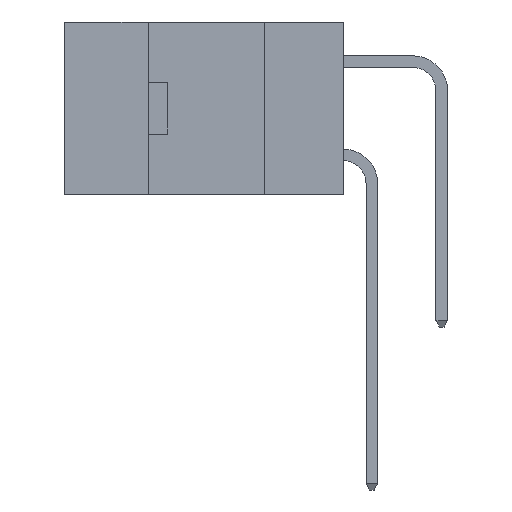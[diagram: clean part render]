
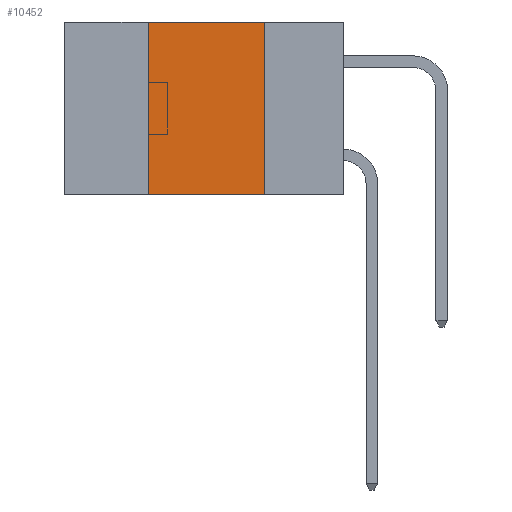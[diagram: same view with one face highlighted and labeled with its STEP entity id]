
A CAD part, left-side view. The second image highlights one B-rep face of the part: STEP entity #10452.
In plain terms, the highlighted planar face has unit normal (-1, 0, 0).
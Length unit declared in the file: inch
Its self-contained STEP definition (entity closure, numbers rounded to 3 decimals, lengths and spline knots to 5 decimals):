
#431 = LINE ( 'NONE', #9070, #17279 ) ;
#852 = EDGE_CURVE ( 'NONE', #18869, #2301, #431, .T. ) ;
#1105 = CARTESIAN_POINT ( 'NONE',  ( 0., 0.17, 0. ) ) ;
#1857 = CARTESIAN_POINT ( 'NONE',  ( 0., 0.42, -0.37 ) ) ;
#2301 = VERTEX_POINT ( 'NONE', #1105 ) ;
#2631 = DIRECTION ( 'NONE',  ( 0., 0., -1. ) ) ;
#4402 = VECTOR ( 'NONE', #2631, 39.37008 ) ;
#4627 = CARTESIAN_POINT ( 'NONE',  ( 0., 0.17, -0.37 ) ) ;
#4772 = ORIENTED_EDGE ( 'NONE', *, *, #12679, .T. ) ;
#5109 = ORIENTED_EDGE ( 'NONE', *, *, #852, .F. ) ;
#7193 = VERTEX_POINT ( 'NONE', #1857 ) ;
#7503 = ORIENTED_EDGE ( 'NONE', *, *, #10421, .F. ) ;
#7547 = DIRECTION ( 'NONE',  ( 0., 0., 1. ) ) ;
#9070 = CARTESIAN_POINT ( 'NONE',  ( 0., 0.6, 0. ) ) ;
#9170 = VECTOR ( 'NONE', #7547, 39.37008 ) ;
#10209 = LINE ( 'NONE', #24585, #4402 ) ;
#10421 = EDGE_CURVE ( 'NONE', #2301, #16166, #10209, .T. ) ;
#10452 = ADVANCED_FACE ( 'NONE', ( #21329 ), #24681, .F. ) ;
#10635 = CARTESIAN_POINT ( 'NONE',  ( 0., 0.42, 0. ) ) ;
#10643 = EDGE_CURVE ( 'NONE', #7193, #18869, #26727, .T. ) ;
#11420 = DIRECTION ( 'NONE',  ( 1., 0., 0. ) ) ;
#11490 = LINE ( 'NONE', #25446, #28327 ) ;
#12679 = EDGE_CURVE ( 'NONE', #7193, #16166, #11490, .T. ) ;
#13891 = AXIS2_PLACEMENT_3D ( 'NONE', #22478, #11420, #26831 ) ;
#16166 = VERTEX_POINT ( 'NONE', #4627 ) ;
#17279 = VECTOR ( 'NONE', #24525, 39.37008 ) ;
#17885 = EDGE_LOOP ( 'NONE', ( #7503, #5109, #23389, #4772 ) ) ;
#18869 = VERTEX_POINT ( 'NONE', #10635 ) ;
#21329 = FACE_OUTER_BOUND ( 'NONE', #17885, .T. ) ;
#22478 = CARTESIAN_POINT ( 'NONE',  ( 0., 0.6, 0. ) ) ;
#23389 = ORIENTED_EDGE ( 'NONE', *, *, #10643, .F. ) ;
#24525 = DIRECTION ( 'NONE',  ( 0., -1., 0. ) ) ;
#24585 = CARTESIAN_POINT ( 'NONE',  ( 0., 0.17, -0.37 ) ) ;
#24681 = PLANE ( 'NONE',  #13891 ) ;
#25180 = CARTESIAN_POINT ( 'NONE',  ( 0., 0.42, -0.37 ) ) ;
#25446 = CARTESIAN_POINT ( 'NONE',  ( 0., 0.6, -0.37 ) ) ;
#26727 = LINE ( 'NONE', #25180, #9170 ) ;
#26831 = DIRECTION ( 'NONE',  ( 0., 0., -1. ) ) ;
#27601 = DIRECTION ( 'NONE',  ( 0., -1., 0. ) ) ;
#28327 = VECTOR ( 'NONE', #27601, 39.37008 ) ;
